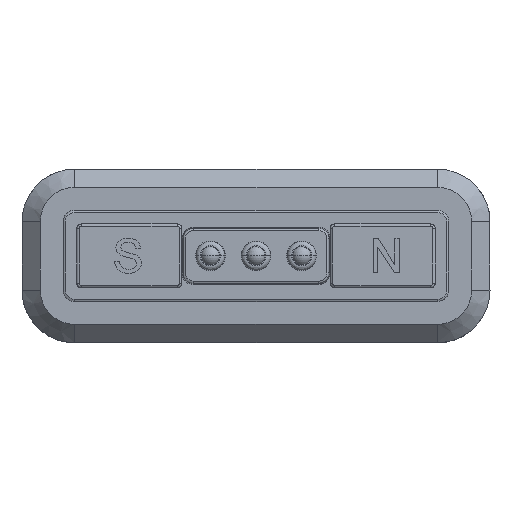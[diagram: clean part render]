
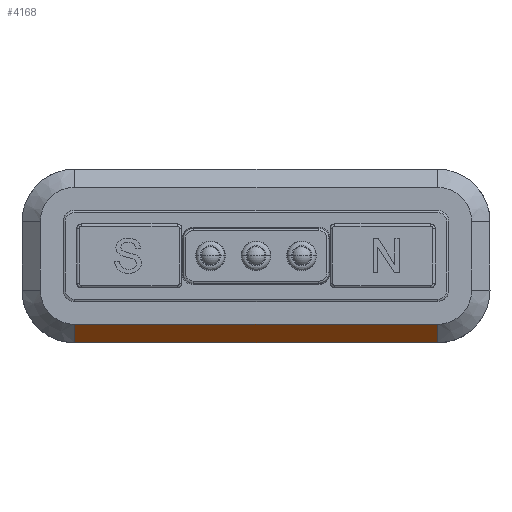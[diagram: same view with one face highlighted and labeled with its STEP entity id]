
A CAD part, top view. The second image highlights one B-rep face of the part: STEP entity #4168.
In plain terms, the highlighted planar face has unit normal (0, -0.707, 0.707).
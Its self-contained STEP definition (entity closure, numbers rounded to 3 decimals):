
#704 = LINE ( 'NONE', #25563, #36116 ) ;
#844 = AXIS2_PLACEMENT_3D ( 'NONE', #15168, #29347, #43506 ) ;
#1005 = PLANE ( 'NONE',  #844 ) ;
#3653 = DIRECTION ( 'NONE',  ( 1., 0., 0. ) ) ;
#4168 = ADVANCED_FACE ( 'NONE', ( #32826 ), #1005, .F. ) ;
#7227 = CARTESIAN_POINT ( 'NONE',  ( -7.95, -3., -0.5 ) ) ;
#8421 = VERTEX_POINT ( 'NONE', #20256 ) ;
#9463 = DIRECTION ( 'NONE',  ( -1., 0., 0. ) ) ;
#11473 = CARTESIAN_POINT ( 'NONE',  ( -7.95, -3., -0.5 ) ) ;
#15168 = CARTESIAN_POINT ( 'NONE',  ( 0., -3.4, -0.9 ) ) ;
#15686 = VECTOR ( 'NONE', #9463, 1000. ) ;
#17165 = EDGE_CURVE ( 'NONE', #23754, #8421, #32624, .T. ) ;
#17462 = VERTEX_POINT ( 'NONE', #43251 ) ;
#18566 = CARTESIAN_POINT ( 'NONE',  ( 7.95, -3., -0.5 ) ) ;
#19606 = EDGE_LOOP ( 'NONE', ( #45616, #38393, #44132, #42126 ) ) ;
#20256 = CARTESIAN_POINT ( 'NONE',  ( -7.95, -3.8, -1.3 ) ) ;
#22922 = EDGE_CURVE ( 'NONE', #37736, #23754, #27133, .T. ) ;
#23754 = VERTEX_POINT ( 'NONE', #7227 ) ;
#24113 = EDGE_CURVE ( 'NONE', #8421, #17462, #45305, .T. ) ;
#25563 = CARTESIAN_POINT ( 'NONE',  ( 7.95, -3.8, -1.3 ) ) ;
#25666 = DIRECTION ( 'NONE',  ( 0., -0.707, -0.707 ) ) ;
#27133 = LINE ( 'NONE', #41304, #15686 ) ;
#28437 = EDGE_CURVE ( 'NONE', #17462, #37736, #704, .T. ) ;
#29347 = DIRECTION ( 'NONE',  ( 0., 0.707, -0.707 ) ) ;
#32624 = LINE ( 'NONE', #11473, #41813 ) ;
#32826 = FACE_OUTER_BOUND ( 'NONE', #19606, .T. ) ;
#35468 = CARTESIAN_POINT ( 'NONE',  ( -7.95, -3.8, -1.3 ) ) ;
#36116 = VECTOR ( 'NONE', #39710, 1000. ) ;
#37736 = VERTEX_POINT ( 'NONE', #18566 ) ;
#38393 = ORIENTED_EDGE ( 'NONE', *, *, #22922, .T. ) ;
#39710 = DIRECTION ( 'NONE',  ( 0., 0.707, 0.707 ) ) ;
#39730 = VECTOR ( 'NONE', #3653, 1000. ) ;
#41304 = CARTESIAN_POINT ( 'NONE',  ( 7.95, -3., -0.5 ) ) ;
#41813 = VECTOR ( 'NONE', #25666, 1000. ) ;
#42126 = ORIENTED_EDGE ( 'NONE', *, *, #24113, .T. ) ;
#43251 = CARTESIAN_POINT ( 'NONE',  ( 7.95, -3.8, -1.3 ) ) ;
#43506 = DIRECTION ( 'NONE',  ( -1., 0., 0. ) ) ;
#44132 = ORIENTED_EDGE ( 'NONE', *, *, #17165, .T. ) ;
#45305 = LINE ( 'NONE', #35468, #39730 ) ;
#45616 = ORIENTED_EDGE ( 'NONE', *, *, #28437, .T. ) ;
